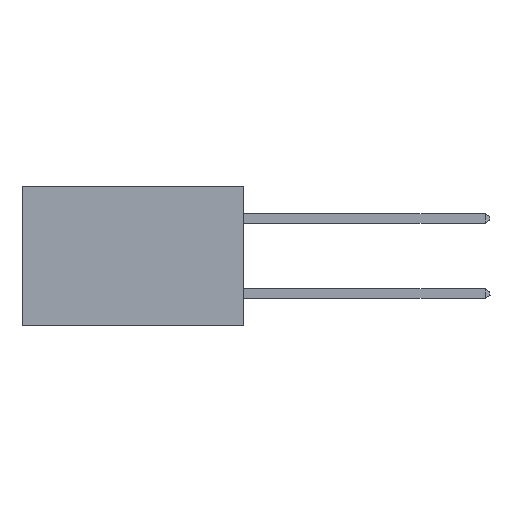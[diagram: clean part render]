
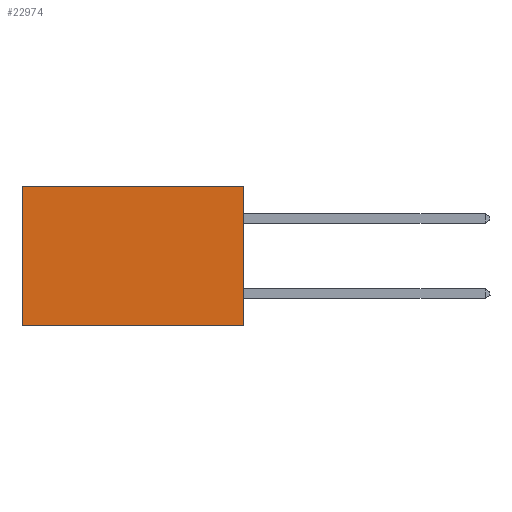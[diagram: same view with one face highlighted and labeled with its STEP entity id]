
A CAD part, left-side view. The second image highlights one B-rep face of the part: STEP entity #22974.
In plain terms, the highlighted planar face has unit normal (-1, 0, 0).
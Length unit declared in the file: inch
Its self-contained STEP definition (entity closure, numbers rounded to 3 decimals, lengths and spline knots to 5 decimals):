
#1402 = AXIS2_PLACEMENT_3D ( 'NONE', #8449, #10741, #26689 ) ;
#2310 = LINE ( 'NONE', #18897, #25374 ) ;
#2463 = EDGE_CURVE ( 'NONE', #21445, #16208, #15311, .T. ) ;
#3040 = LINE ( 'NONE', #20648, #8547 ) ;
#5715 = EDGE_CURVE ( 'NONE', #18136, #21445, #13213, .T. ) ;
#5825 = ORIENTED_EDGE ( 'NONE', *, *, #5715, .F. ) ;
#6146 = EDGE_CURVE ( 'NONE', #18136, #7431, #2310, .T. ) ;
#6392 = VECTOR ( 'NONE', #16895, 39.37008 ) ;
#7361 = CARTESIAN_POINT ( 'NONE',  ( 0.277, 0., -0.37 ) ) ;
#7431 = VERTEX_POINT ( 'NONE', #10553 ) ;
#8449 = CARTESIAN_POINT ( 'NONE',  ( 0.277, 0., -0.37 ) ) ;
#8547 = VECTOR ( 'NONE', #20734, 39.37008 ) ;
#10227 = DIRECTION ( 'NONE',  ( 0., 1., 0. ) ) ;
#10245 = CARTESIAN_POINT ( 'NONE',  ( 0.277, 0.59, -0.37 ) ) ;
#10553 = CARTESIAN_POINT ( 'NONE',  ( 0.277, 0.59, 0. ) ) ;
#10741 = DIRECTION ( 'NONE',  ( 1., 0., 0. ) ) ;
#12254 = ORIENTED_EDGE ( 'NONE', *, *, #2463, .F. ) ;
#12359 = CARTESIAN_POINT ( 'NONE',  ( 0.277, 0., 0. ) ) ;
#12499 = EDGE_LOOP ( 'NONE', ( #17732, #12254, #5825, #21852 ) ) ;
#13213 = LINE ( 'NONE', #17069, #6392 ) ;
#14359 = FACE_OUTER_BOUND ( 'NONE', #12499, .T. ) ;
#15311 = LINE ( 'NONE', #7361, #16747 ) ;
#16208 = VERTEX_POINT ( 'NONE', #10245 ) ;
#16747 = VECTOR ( 'NONE', #10227, 39.37008 ) ;
#16895 = DIRECTION ( 'NONE',  ( 0., 0., -1. ) ) ;
#17069 = CARTESIAN_POINT ( 'NONE',  ( 0.277, 0., -0.37 ) ) ;
#17732 = ORIENTED_EDGE ( 'NONE', *, *, #29099, .T. ) ;
#18136 = VERTEX_POINT ( 'NONE', #12359 ) ;
#18872 = CARTESIAN_POINT ( 'NONE',  ( 0.277, 0., -0.37 ) ) ;
#18897 = CARTESIAN_POINT ( 'NONE',  ( 0.277, 0., 0. ) ) ;
#19537 = DIRECTION ( 'NONE',  ( 0., 1., 0. ) ) ;
#20648 = CARTESIAN_POINT ( 'NONE',  ( 0.277, 0.59, -0.37 ) ) ;
#20734 = DIRECTION ( 'NONE',  ( 0., 0., -1. ) ) ;
#21445 = VERTEX_POINT ( 'NONE', #18872 ) ;
#21852 = ORIENTED_EDGE ( 'NONE', *, *, #6146, .T. ) ;
#22183 = PLANE ( 'NONE',  #1402 ) ;
#22974 = ADVANCED_FACE ( 'NONE', ( #14359 ), #22183, .F. ) ;
#25374 = VECTOR ( 'NONE', #19537, 39.37008 ) ;
#26689 = DIRECTION ( 'NONE',  ( 0., 0., -1. ) ) ;
#29099 = EDGE_CURVE ( 'NONE', #7431, #16208, #3040, .T. ) ;
